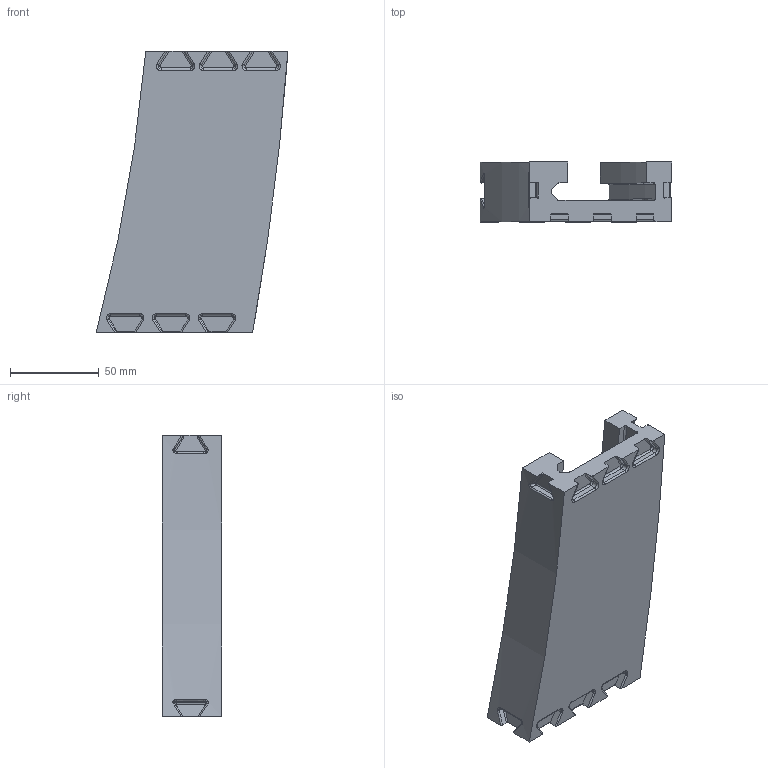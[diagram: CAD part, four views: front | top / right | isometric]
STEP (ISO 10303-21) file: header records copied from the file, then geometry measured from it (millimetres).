
FILE_DESCRIPTION(/* description */ (''),/* implementation_level */ '2;1');
FILE_NAME(/* name */ 'freeman1337-speedloader-middle-v4-engraved.step',/* time_stamp */ '2021-09-03T15:15:41-07:00',/* author */ (''),/* organization */ (''),/* preprocessor_version */ 'ST-DEVELOPER v18.1',/* originating_system */ 'Autodesk Translation Framework v10.10.0.1391',/* authorisation */ '');
FILE_SCHEMA (('AUTOMOTIVE_DESIGN { 1 0 10303 214 3 1 1 }'));
Length unit declared in the file: millimetre
Products named in the file (1): loader-middle
Bounding box: 108.23 x 33.62 x 158.74 mm (x, y, z)
Volume: 262197.5 mm3; surface area: 53697.8 mm2
Topology: 1 solids, 1 shells, 1012 faces, 2726 edges, 1784 vertices
Faces by surface type: plane 476, bspline 434, cylinder 81, torus 21
Entity records: 36236 total; most frequent: CARTESIAN_POINT 13615, ORIENTED_EDGE 5444, DIRECTION 3283, EDGE_CURVE 2722, VERTEX_POINT 1784, LINE 1647, VECTOR 1647, EDGE_LOOP 1084
